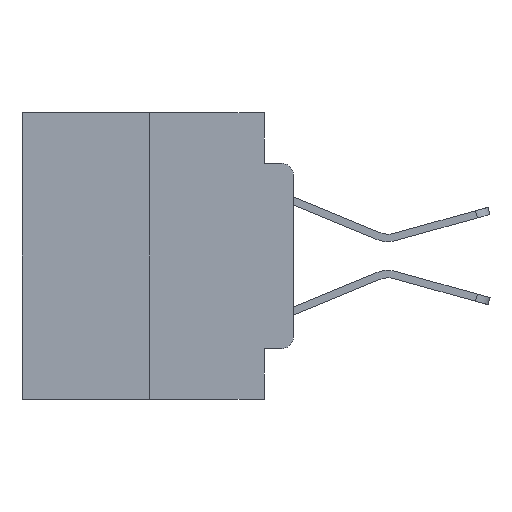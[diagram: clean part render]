
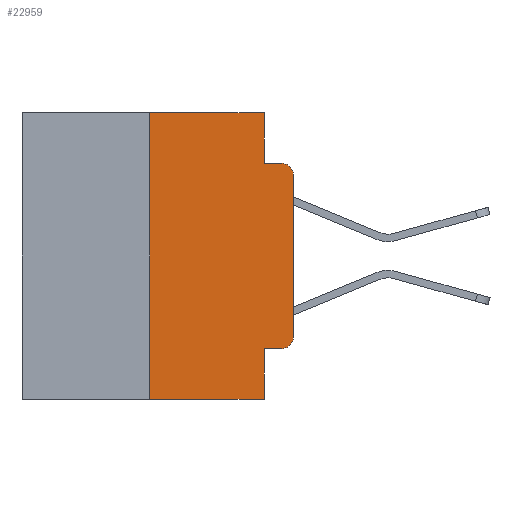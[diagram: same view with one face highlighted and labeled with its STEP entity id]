
A CAD part, left-side view. The second image highlights one B-rep face of the part: STEP entity #22959.
In plain terms, the highlighted planar face has unit normal (-1, 0, 0).
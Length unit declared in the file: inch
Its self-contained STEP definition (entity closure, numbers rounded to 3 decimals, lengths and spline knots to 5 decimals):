
#402 = AXIS2_PLACEMENT_3D ( 'NONE', #11123, #13101, #2716 ) ;
#769 = EDGE_CURVE ( 'NONE', #6550, #7935, #26523, .T. ) ;
#859 = DIRECTION ( 'NONE',  ( 0., 0., -1. ) ) ;
#975 = VECTOR ( 'NONE', #4603, 39.37008 ) ;
#1138 = AXIS2_PLACEMENT_3D ( 'NONE', #14845, #5961, #23245 ) ;
#1245 = CARTESIAN_POINT ( 'NONE',  ( 0., 0.051, -0.5 ) ) ;
#1348 = CIRCLE ( 'NONE', #14506, 0.02 ) ;
#1425 = EDGE_CURVE ( 'NONE', #25867, #23968, #20509, .T. ) ;
#1798 = VERTEX_POINT ( 'NONE', #1245 ) ;
#1844 = CARTESIAN_POINT ( 'NONE',  ( 0., 0.051, -0.4115 ) ) ;
#1862 = VECTOR ( 'NONE', #22037, 39.37008 ) ;
#2525 = LINE ( 'NONE', #2625, #9805 ) ;
#2625 = CARTESIAN_POINT ( 'NONE',  ( 0., 0.051, 0. ) ) ;
#2716 = DIRECTION ( 'NONE',  ( 0., 0., -1. ) ) ;
#3291 = CARTESIAN_POINT ( 'NONE',  ( 0., 0.02, -0.4115 ) ) ;
#3611 = CARTESIAN_POINT ( 'NONE',  ( 0., 0.02, -0.0885 ) ) ;
#4271 = ORIENTED_EDGE ( 'NONE', *, *, #769, .F. ) ;
#4405 = ORIENTED_EDGE ( 'NONE', *, *, #27497, .T. ) ;
#4451 = EDGE_CURVE ( 'NONE', #25571, #1798, #26779, .T. ) ;
#4536 = EDGE_CURVE ( 'NONE', #23968, #6550, #2525, .T. ) ;
#4603 = DIRECTION ( 'NONE',  ( 0., 0., 1. ) ) ;
#5155 = ORIENTED_EDGE ( 'NONE', *, *, #12262, .T. ) ;
#5420 = CARTESIAN_POINT ( 'NONE',  ( 0., 0.051, -0.4115 ) ) ;
#5697 = EDGE_LOOP ( 'NONE', ( #4405, #24497, #4271, #9022, #14247, #23920, #5155, #18299, #21496, #12192 ) ) ;
#5961 = DIRECTION ( 'NONE',  ( 1., 0., 0. ) ) ;
#6021 = CARTESIAN_POINT ( 'NONE',  ( 0., 0.473, 0. ) ) ;
#6459 = VERTEX_POINT ( 'NONE', #3291 ) ;
#6550 = VERTEX_POINT ( 'NONE', #16468 ) ;
#6846 = CARTESIAN_POINT ( 'NONE',  ( 0., 0.25, 0. ) ) ;
#7687 = LINE ( 'NONE', #6846, #21314 ) ;
#7849 = DIRECTION ( 'NONE',  ( 0., -1., 0. ) ) ;
#7935 = VERTEX_POINT ( 'NONE', #3611 ) ;
#8918 = CARTESIAN_POINT ( 'NONE',  ( 0., 0.051, 0. ) ) ;
#9022 = ORIENTED_EDGE ( 'NONE', *, *, #4536, .F. ) ;
#9673 = CARTESIAN_POINT ( 'NONE',  ( 0., 0.051, 0. ) ) ;
#9786 = CARTESIAN_POINT ( 'NONE',  ( 0., 0.02, -0.3915 ) ) ;
#9805 = VECTOR ( 'NONE', #859, 39.37008 ) ;
#9834 = VECTOR ( 'NONE', #7849, 39.37008 ) ;
#10739 = EDGE_CURVE ( 'NONE', #25571, #6459, #25881, .T. ) ;
#11123 = CARTESIAN_POINT ( 'NONE',  ( 0., 0.02, -0.1085 ) ) ;
#11156 = CIRCLE ( 'NONE', #402, 0.02 ) ;
#11228 = VECTOR ( 'NONE', #23215, 39.37008 ) ;
#11911 = DIRECTION ( 'NONE',  ( 0., 0., -1. ) ) ;
#12192 = ORIENTED_EDGE ( 'NONE', *, *, #26848, .T. ) ;
#12262 = EDGE_CURVE ( 'NONE', #24824, #1798, #15487, .T. ) ;
#13101 = DIRECTION ( 'NONE',  ( -1., 0., 0. ) ) ;
#13312 = CARTESIAN_POINT ( 'NONE',  ( 0., 0., -0.3915 ) ) ;
#13329 = DIRECTION ( 'NONE',  ( 0., 0., 1. ) ) ;
#14247 = ORIENTED_EDGE ( 'NONE', *, *, #1425, .F. ) ;
#14506 = AXIS2_PLACEMENT_3D ( 'NONE', #9786, #24387, #11911 ) ;
#14845 = CARTESIAN_POINT ( 'NONE',  ( 0., 0.473, 0. ) ) ;
#14849 = VECTOR ( 'NONE', #27370, 39.37008 ) ;
#15487 = LINE ( 'NONE', #22827, #9834 ) ;
#16468 = CARTESIAN_POINT ( 'NONE',  ( 0., 0.051, -0.0885 ) ) ;
#16620 = CARTESIAN_POINT ( 'NONE',  ( 0., 0.25, 0. ) ) ;
#17412 = CARTESIAN_POINT ( 'NONE',  ( 0., 0., -0.1085 ) ) ;
#17962 = VERTEX_POINT ( 'NONE', #17412 ) ;
#18024 = EDGE_CURVE ( 'NONE', #24824, #25867, #7687, .T. ) ;
#18299 = ORIENTED_EDGE ( 'NONE', *, *, #4451, .F. ) ;
#18467 = FACE_OUTER_BOUND ( 'NONE', #5697, .T. ) ;
#19233 = LINE ( 'NONE', #25844, #975 ) ;
#20509 = LINE ( 'NONE', #6021, #14849 ) ;
#20895 = VECTOR ( 'NONE', #23681, 39.37008 ) ;
#21314 = VECTOR ( 'NONE', #13329, 39.37008 ) ;
#21496 = ORIENTED_EDGE ( 'NONE', *, *, #10739, .T. ) ;
#22037 = DIRECTION ( 'NONE',  ( 0., 0., -1. ) ) ;
#22544 = EDGE_CURVE ( 'NONE', #17962, #7935, #11156, .T. ) ;
#22827 = CARTESIAN_POINT ( 'NONE',  ( 0., 0.473, -0.5 ) ) ;
#22959 = ADVANCED_FACE ( 'NONE', ( #18467 ), #23149, .F. ) ;
#23149 = PLANE ( 'NONE',  #1138 ) ;
#23215 = DIRECTION ( 'NONE',  ( 0., -1., 0. ) ) ;
#23245 = DIRECTION ( 'NONE',  ( 0., 0., -1. ) ) ;
#23681 = DIRECTION ( 'NONE',  ( 0., -1., 0. ) ) ;
#23920 = ORIENTED_EDGE ( 'NONE', *, *, #18024, .F. ) ;
#23968 = VERTEX_POINT ( 'NONE', #9673 ) ;
#24108 = CARTESIAN_POINT ( 'NONE',  ( 0., 0.25, -0.5 ) ) ;
#24387 = DIRECTION ( 'NONE',  ( -1., 0., 0. ) ) ;
#24497 = ORIENTED_EDGE ( 'NONE', *, *, #22544, .T. ) ;
#24658 = VERTEX_POINT ( 'NONE', #13312 ) ;
#24824 = VERTEX_POINT ( 'NONE', #24108 ) ;
#25571 = VERTEX_POINT ( 'NONE', #5420 ) ;
#25714 = CARTESIAN_POINT ( 'NONE',  ( 0., 0.051, -0.0885 ) ) ;
#25844 = CARTESIAN_POINT ( 'NONE',  ( 0., 0., 0. ) ) ;
#25867 = VERTEX_POINT ( 'NONE', #16620 ) ;
#25881 = LINE ( 'NONE', #1844, #11228 ) ;
#26523 = LINE ( 'NONE', #25714, #20895 ) ;
#26779 = LINE ( 'NONE', #8918, #1862 ) ;
#26848 = EDGE_CURVE ( 'NONE', #6459, #24658, #1348, .T. ) ;
#27370 = DIRECTION ( 'NONE',  ( 0., -1., 0. ) ) ;
#27497 = EDGE_CURVE ( 'NONE', #24658, #17962, #19233, .T. ) ;
